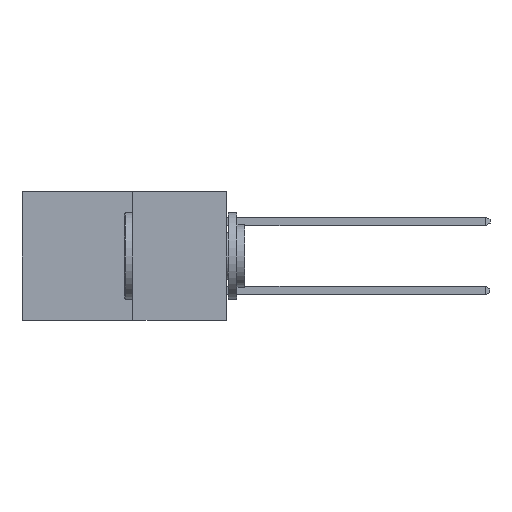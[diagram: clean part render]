
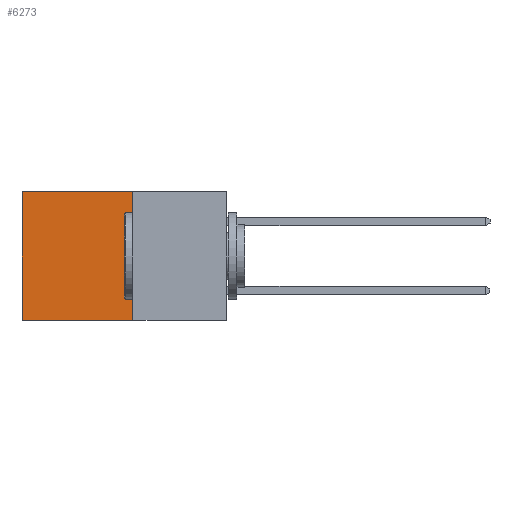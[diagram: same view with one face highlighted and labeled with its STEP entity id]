
A CAD part, left-side view. The second image highlights one B-rep face of the part: STEP entity #6273.
In plain terms, the highlighted planar face has unit normal (-1, 0, 0).
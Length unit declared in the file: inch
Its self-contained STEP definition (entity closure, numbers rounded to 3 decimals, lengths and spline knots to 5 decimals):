
#698 = AXIS2_PLACEMENT_3D ( 'NONE', #12526, #19244, #5768 ) ;
#1231 = VECTOR ( 'NONE', #1376, 39.37008 ) ;
#1376 = DIRECTION ( 'NONE',  ( 0., 0., -1. ) ) ;
#1713 = LINE ( 'NONE', #20588, #18310 ) ;
#2533 = DIRECTION ( 'NONE',  ( 0., 0., -1. ) ) ;
#2696 = CARTESIAN_POINT ( 'NONE',  ( 0.277, 0.27, 0. ) ) ;
#3831 = ORIENTED_EDGE ( 'NONE', *, *, #12556, .T. ) ;
#3969 = ORIENTED_EDGE ( 'NONE', *, *, #9086, .F. ) ;
#4970 = CARTESIAN_POINT ( 'NONE',  ( 0.277, 0.59, -0.37 ) ) ;
#5743 = LINE ( 'NONE', #22849, #6475 ) ;
#5760 = VECTOR ( 'NONE', #12623, 39.37008 ) ;
#5768 = DIRECTION ( 'NONE',  ( 0., 0., -1. ) ) ;
#6273 = ADVANCED_FACE ( 'NONE', ( #13734 ), #17013, .F. ) ;
#6475 = VECTOR ( 'NONE', #7252, 39.37008 ) ;
#6489 = LINE ( 'NONE', #10370, #5760 ) ;
#7158 = CARTESIAN_POINT ( 'NONE',  ( 0.277, 0.27, -0.37 ) ) ;
#7252 = DIRECTION ( 'NONE',  ( 0., 1., 0. ) ) ;
#7255 = CARTESIAN_POINT ( 'NONE',  ( 0.277, 0.59, 0. ) ) ;
#9086 = EDGE_CURVE ( 'NONE', #22332, #16910, #5743, .T. ) ;
#10370 = CARTESIAN_POINT ( 'NONE',  ( 0.277, 0.27, 0. ) ) ;
#10427 = EDGE_CURVE ( 'NONE', #13561, #22332, #1713, .T. ) ;
#11207 = LINE ( 'NONE', #28103, #1231 ) ;
#12526 = CARTESIAN_POINT ( 'NONE',  ( 0.277, 0.27, -0.37 ) ) ;
#12556 = EDGE_CURVE ( 'NONE', #19015, #16910, #11207, .T. ) ;
#12623 = DIRECTION ( 'NONE',  ( 0., 1., 0. ) ) ;
#13561 = VERTEX_POINT ( 'NONE', #2696 ) ;
#13734 = FACE_OUTER_BOUND ( 'NONE', #16724, .T. ) ;
#16724 = EDGE_LOOP ( 'NONE', ( #3831, #3969, #18273, #27549 ) ) ;
#16910 = VERTEX_POINT ( 'NONE', #4970 ) ;
#17013 = PLANE ( 'NONE',  #698 ) ;
#18273 = ORIENTED_EDGE ( 'NONE', *, *, #10427, .F. ) ;
#18310 = VECTOR ( 'NONE', #2533, 39.37008 ) ;
#19015 = VERTEX_POINT ( 'NONE', #7255 ) ;
#19244 = DIRECTION ( 'NONE',  ( 1., 0., 0. ) ) ;
#20588 = CARTESIAN_POINT ( 'NONE',  ( 0.277, 0.27, -0.37 ) ) ;
#21364 = EDGE_CURVE ( 'NONE', #13561, #19015, #6489, .T. ) ;
#22332 = VERTEX_POINT ( 'NONE', #7158 ) ;
#22849 = CARTESIAN_POINT ( 'NONE',  ( 0.277, 0.27, -0.37 ) ) ;
#27549 = ORIENTED_EDGE ( 'NONE', *, *, #21364, .T. ) ;
#28103 = CARTESIAN_POINT ( 'NONE',  ( 0.277, 0.59, -0.37 ) ) ;
